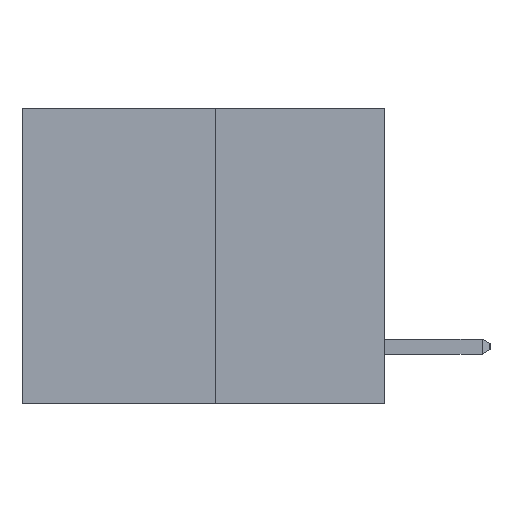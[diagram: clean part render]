
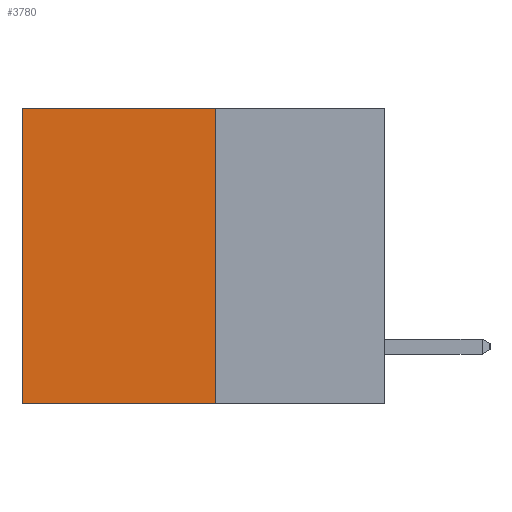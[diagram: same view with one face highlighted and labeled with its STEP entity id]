
A CAD part, left-side view. The second image highlights one B-rep face of the part: STEP entity #3780.
In plain terms, the highlighted planar face has unit normal (-1, 0, 0).
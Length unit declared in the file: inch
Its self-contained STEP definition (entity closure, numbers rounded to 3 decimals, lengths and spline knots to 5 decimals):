
#153 = AXIS2_PLACEMENT_3D ( 'NONE', #8067, #1928, #1985 ) ;
#718 = ORIENTED_EDGE ( 'NONE', *, *, #6288, .T. ) ;
#991 = LINE ( 'NONE', #8705, #1462 ) ;
#1462 = VECTOR ( 'NONE', #4121, 39.37008 ) ;
#1621 = VERTEX_POINT ( 'NONE', #9382 ) ;
#1928 = DIRECTION ( 'NONE',  ( 1., 0., 0. ) ) ;
#1985 = DIRECTION ( 'NONE',  ( 0., 0., -1. ) ) ;
#2067 = DIRECTION ( 'NONE',  ( 0., 0., -1. ) ) ;
#2087 = VERTEX_POINT ( 'NONE', #6100 ) ;
#2230 = FACE_OUTER_BOUND ( 'NONE', #8469, .T. ) ;
#2508 = CARTESIAN_POINT ( 'NONE',  ( 0.3165, 0.6, -0.49 ) ) ;
#2548 = EDGE_CURVE ( 'NONE', #2087, #6733, #991, .T. ) ;
#2760 = PLANE ( 'NONE',  #153 ) ;
#3107 = ORIENTED_EDGE ( 'NONE', *, *, #6582, .F. ) ;
#3145 = DIRECTION ( 'NONE',  ( 0., 0., -1. ) ) ;
#3343 = ORIENTED_EDGE ( 'NONE', *, *, #2548, .T. ) ;
#3780 = ADVANCED_FACE ( 'NONE', ( #2230 ), #2760, .F. ) ;
#3846 = VECTOR ( 'NONE', #6003, 39.37008 ) ;
#3863 = CARTESIAN_POINT ( 'NONE',  ( 0.3165, 0.28, -0.49 ) ) ;
#4121 = DIRECTION ( 'NONE',  ( 0., 1., 0. ) ) ;
#4231 = CARTESIAN_POINT ( 'NONE',  ( 0.3165, 0.28, -0.49 ) ) ;
#4302 = LINE ( 'NONE', #6722, #3846 ) ;
#5630 = VECTOR ( 'NONE', #3145, 39.37008 ) ;
#5949 = LINE ( 'NONE', #4231, #7988 ) ;
#6003 = DIRECTION ( 'NONE',  ( 0., 1., 0. ) ) ;
#6100 = CARTESIAN_POINT ( 'NONE',  ( 0.3165, 0.28, 0. ) ) ;
#6288 = EDGE_CURVE ( 'NONE', #6733, #1621, #8023, .T. ) ;
#6582 = EDGE_CURVE ( 'NONE', #9722, #1621, #4302, .T. ) ;
#6722 = CARTESIAN_POINT ( 'NONE',  ( 0.3165, 0.28, -0.49 ) ) ;
#6733 = VERTEX_POINT ( 'NONE', #7648 ) ;
#7648 = CARTESIAN_POINT ( 'NONE',  ( 0.3165, 0.6, 0. ) ) ;
#7988 = VECTOR ( 'NONE', #2067, 39.37008 ) ;
#8023 = LINE ( 'NONE', #2508, #5630 ) ;
#8067 = CARTESIAN_POINT ( 'NONE',  ( 0.3165, 0.28, -0.49 ) ) ;
#8092 = EDGE_CURVE ( 'NONE', #2087, #9722, #5949, .T. ) ;
#8469 = EDGE_LOOP ( 'NONE', ( #718, #3107, #8513, #3343 ) ) ;
#8513 = ORIENTED_EDGE ( 'NONE', *, *, #8092, .F. ) ;
#8705 = CARTESIAN_POINT ( 'NONE',  ( 0.3165, 0.28, 0. ) ) ;
#9382 = CARTESIAN_POINT ( 'NONE',  ( 0.3165, 0.6, -0.49 ) ) ;
#9722 = VERTEX_POINT ( 'NONE', #3863 ) ;
